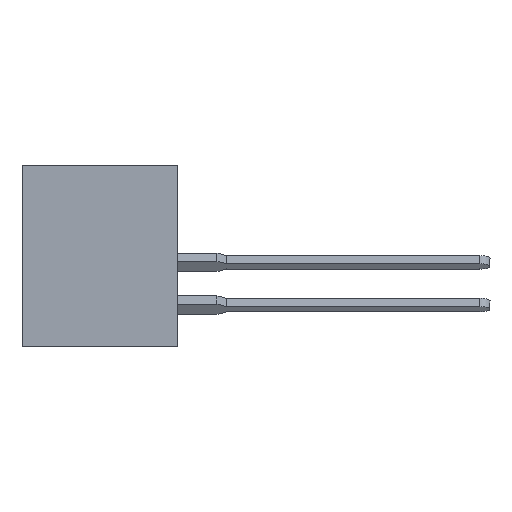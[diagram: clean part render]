
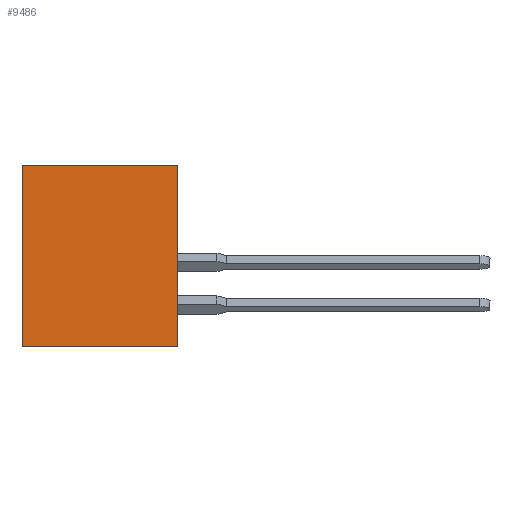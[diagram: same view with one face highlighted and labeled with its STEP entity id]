
A CAD part, left-side view. The second image highlights one B-rep face of the part: STEP entity #9486.
In plain terms, the highlighted planar face has unit normal (-1, 0, 0).
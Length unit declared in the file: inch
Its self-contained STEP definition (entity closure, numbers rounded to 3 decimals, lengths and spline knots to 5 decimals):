
#28 = EDGE_CURVE ( 'NONE', #5858, #7881, #2223, .T. ) ;
#302 = EDGE_CURVE ( 'NONE', #5858, #1423, #13990, .T. ) ;
#527 = LINE ( 'NONE', #13206, #903 ) ;
#903 = VECTOR ( 'NONE', #8219, 39.37008 ) ;
#1423 = VERTEX_POINT ( 'NONE', #15052 ) ;
#1566 = DIRECTION ( 'NONE',  ( 0., 0., 1. ) ) ;
#1976 = VERTEX_POINT ( 'NONE', #13565 ) ;
#2072 = CARTESIAN_POINT ( 'NONE',  ( 0., 0.453, -0.531 ) ) ;
#2223 = LINE ( 'NONE', #4099, #14563 ) ;
#4099 = CARTESIAN_POINT ( 'NONE',  ( 0., 0.453, 0. ) ) ;
#5289 = AXIS2_PLACEMENT_3D ( 'NONE', #5299, #6534, #7742 ) ;
#5299 = CARTESIAN_POINT ( 'NONE',  ( 0., 0.453, 0. ) ) ;
#5634 = VECTOR ( 'NONE', #5804, 39.37008 ) ;
#5804 = DIRECTION ( 'NONE',  ( 0., -1., 0. ) ) ;
#5858 = VERTEX_POINT ( 'NONE', #12223 ) ;
#6534 = DIRECTION ( 'NONE',  ( 1., 0., 0. ) ) ;
#6564 = FACE_OUTER_BOUND ( 'NONE', #8473, .T. ) ;
#7742 = DIRECTION ( 'NONE',  ( 0., 0., -1. ) ) ;
#7881 = VERTEX_POINT ( 'NONE', #11359 ) ;
#8191 = EDGE_CURVE ( 'NONE', #1423, #1976, #527, .T. ) ;
#8219 = DIRECTION ( 'NONE',  ( 0., 0., 1. ) ) ;
#8473 = EDGE_LOOP ( 'NONE', ( #14974, #8643, #9761, #12536 ) ) ;
#8643 = ORIENTED_EDGE ( 'NONE', *, *, #12279, .F. ) ;
#9486 = ADVANCED_FACE ( 'NONE', ( #6564 ), #10244, .F. ) ;
#9761 = ORIENTED_EDGE ( 'NONE', *, *, #28, .F. ) ;
#10244 = PLANE ( 'NONE',  #5289 ) ;
#10668 = DIRECTION ( 'NONE',  ( 0., -1., 0. ) ) ;
#10777 = CARTESIAN_POINT ( 'NONE',  ( 0., 0.453, 0. ) ) ;
#11359 = CARTESIAN_POINT ( 'NONE',  ( 0., 0.453, 0. ) ) ;
#12223 = CARTESIAN_POINT ( 'NONE',  ( 0., 0.453, -0.531 ) ) ;
#12279 = EDGE_CURVE ( 'NONE', #7881, #1976, #14383, .T. ) ;
#12313 = VECTOR ( 'NONE', #10668, 39.37008 ) ;
#12536 = ORIENTED_EDGE ( 'NONE', *, *, #302, .T. ) ;
#13206 = CARTESIAN_POINT ( 'NONE',  ( 0., 0., 0. ) ) ;
#13565 = CARTESIAN_POINT ( 'NONE',  ( 0., 0., 0. ) ) ;
#13990 = LINE ( 'NONE', #2072, #5634 ) ;
#14383 = LINE ( 'NONE', #10777, #12313 ) ;
#14563 = VECTOR ( 'NONE', #1566, 39.37008 ) ;
#14974 = ORIENTED_EDGE ( 'NONE', *, *, #8191, .T. ) ;
#15052 = CARTESIAN_POINT ( 'NONE',  ( 0., 0., -0.531 ) ) ;
